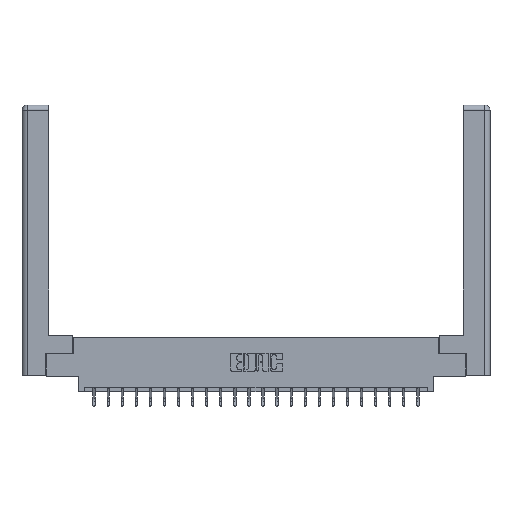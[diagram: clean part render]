
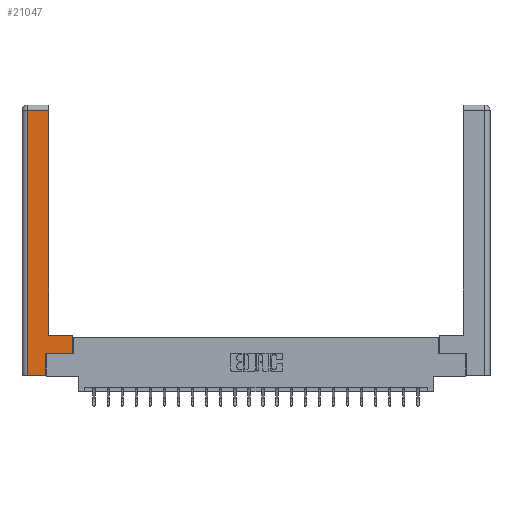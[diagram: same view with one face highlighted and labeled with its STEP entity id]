
A CAD part, top view. The second image highlights one B-rep face of the part: STEP entity #21047.
In plain terms, the highlighted planar face has unit normal (0, 0, 1).
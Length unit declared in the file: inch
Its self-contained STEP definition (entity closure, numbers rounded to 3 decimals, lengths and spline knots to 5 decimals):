
#773 = CARTESIAN_POINT ( 'NONE',  ( 0.0615, 0., 0. ) ) ;
#780 = ORIENTED_EDGE ( 'NONE', *, *, #12430, .T. ) ;
#1169 = DIRECTION ( 'NONE',  ( 0., 1., 0. ) ) ;
#1950 = VERTEX_POINT ( 'NONE', #4467 ) ;
#2144 = LINE ( 'NONE', #4734, #14895 ) ;
#2428 = EDGE_CURVE ( 'NONE', #11422, #19832, #10936, .T. ) ;
#3939 = EDGE_CURVE ( 'NONE', #20765, #15186, #18033, .T. ) ;
#4144 = FACE_OUTER_BOUND ( 'NONE', #19279, .T. ) ;
#4195 = ORIENTED_EDGE ( 'NONE', *, *, #19526, .T. ) ;
#4467 = CARTESIAN_POINT ( 'NONE',  ( 0.295, 2.94, 0. ) ) ;
#4545 = CARTESIAN_POINT ( 'NONE',  ( 0.565, 0.245, 0. ) ) ;
#4734 = CARTESIAN_POINT ( 'NONE',  ( 0.295, 3., 0. ) ) ;
#4741 = VECTOR ( 'NONE', #18252, 39.37008 ) ;
#4781 = CARTESIAN_POINT ( 'NONE',  ( 0., 0., 0. ) ) ;
#5537 = CARTESIAN_POINT ( 'NONE',  ( 0.565, 0.45, 0. ) ) ;
#5594 = DIRECTION ( 'NONE',  ( 1., 0., 0. ) ) ;
#5794 = DIRECTION ( 'NONE',  ( -1., 0., 0. ) ) ;
#5872 = EDGE_CURVE ( 'NONE', #15186, #10051, #22398, .T. ) ;
#5995 = VERTEX_POINT ( 'NONE', #10482 ) ;
#6660 = DIRECTION ( 'NONE',  ( 0., 0., -1. ) ) ;
#6691 = CARTESIAN_POINT ( 'NONE',  ( 0.565, 0.45, 0. ) ) ;
#7129 = EDGE_CURVE ( 'NONE', #5995, #7491, #17697, .T. ) ;
#7416 = EDGE_CURVE ( 'NONE', #1950, #5995, #10201, .T. ) ;
#7491 = VERTEX_POINT ( 'NONE', #11588 ) ;
#7968 = DIRECTION ( 'NONE',  ( 0., -1., 0. ) ) ;
#8718 = DIRECTION ( 'NONE',  ( -1., 0., 0. ) ) ;
#9488 = VECTOR ( 'NONE', #8718, 39.37008 ) ;
#9900 = CARTESIAN_POINT ( 'NONE',  ( 0.265, 0., 0. ) ) ;
#10051 = VERTEX_POINT ( 'NONE', #4545 ) ;
#10201 = LINE ( 'NONE', #21926, #16247 ) ;
#10288 = VECTOR ( 'NONE', #5594, 39.37008 ) ;
#10482 = CARTESIAN_POINT ( 'NONE',  ( 0.0615, 2.94, 0. ) ) ;
#10936 = LINE ( 'NONE', #23817, #9488 ) ;
#11086 = CARTESIAN_POINT ( 'NONE',  ( 0.295, 0.45, 0. ) ) ;
#11422 = VERTEX_POINT ( 'NONE', #5537 ) ;
#11588 = CARTESIAN_POINT ( 'NONE',  ( 0.0615, 0., 0. ) ) ;
#11946 = ORIENTED_EDGE ( 'NONE', *, *, #20375, .T. ) ;
#12166 = VECTOR ( 'NONE', #17297, 39.37008 ) ;
#12208 = DIRECTION ( 'NONE',  ( -1., 0., 0. ) ) ;
#12430 = EDGE_CURVE ( 'NONE', #7491, #20765, #21692, .T. ) ;
#12675 = CARTESIAN_POINT ( 'NONE',  ( 0.265, 0.245, 0. ) ) ;
#13048 = CARTESIAN_POINT ( 'NONE',  ( 0.265, 0., 0. ) ) ;
#13654 = CARTESIAN_POINT ( 'NONE',  ( 0.265, 0.245, 0. ) ) ;
#13829 = ORIENTED_EDGE ( 'NONE', *, *, #5872, .T. ) ;
#14895 = VECTOR ( 'NONE', #19420, 39.37008 ) ;
#15186 = VERTEX_POINT ( 'NONE', #13654 ) ;
#16231 = ORIENTED_EDGE ( 'NONE', *, *, #2428, .T. ) ;
#16247 = VECTOR ( 'NONE', #5794, 39.37008 ) ;
#17297 = DIRECTION ( 'NONE',  ( 1., 0., 0. ) ) ;
#17336 = ORIENTED_EDGE ( 'NONE', *, *, #3939, .T. ) ;
#17697 = LINE ( 'NONE', #773, #23493 ) ;
#18033 = LINE ( 'NONE', #12675, #4741 ) ;
#18252 = DIRECTION ( 'NONE',  ( 0., 1., 0. ) ) ;
#18317 = AXIS2_PLACEMENT_3D ( 'NONE', #4781, #6660, #12208 ) ;
#19279 = EDGE_LOOP ( 'NONE', ( #11946, #23940, #22017, #780, #17336, #13829, #4195, #16231 ) ) ;
#19420 = DIRECTION ( 'NONE',  ( 0., 1., 0. ) ) ;
#19526 = EDGE_CURVE ( 'NONE', #10051, #11422, #22159, .T. ) ;
#19832 = VERTEX_POINT ( 'NONE', #11086 ) ;
#20375 = EDGE_CURVE ( 'NONE', #19832, #1950, #2144, .T. ) ;
#20765 = VERTEX_POINT ( 'NONE', #13048 ) ;
#21047 = ADVANCED_FACE ( 'NONE', ( #4144 ), #21417, .F. ) ;
#21417 = PLANE ( 'NONE',  #18317 ) ;
#21692 = LINE ( 'NONE', #9900, #12166 ) ;
#21926 = CARTESIAN_POINT ( 'NONE',  ( 0.0615, 2.94, 0. ) ) ;
#22017 = ORIENTED_EDGE ( 'NONE', *, *, #7129, .T. ) ;
#22159 = LINE ( 'NONE', #6691, #23583 ) ;
#22270 = CARTESIAN_POINT ( 'NONE',  ( 0.565, 0.245, 0. ) ) ;
#22398 = LINE ( 'NONE', #22270, #10288 ) ;
#23493 = VECTOR ( 'NONE', #7968, 39.37008 ) ;
#23583 = VECTOR ( 'NONE', #1169, 39.37008 ) ;
#23817 = CARTESIAN_POINT ( 'NONE',  ( 0.295, 0.45, 0. ) ) ;
#23940 = ORIENTED_EDGE ( 'NONE', *, *, #7416, .T. ) ;
